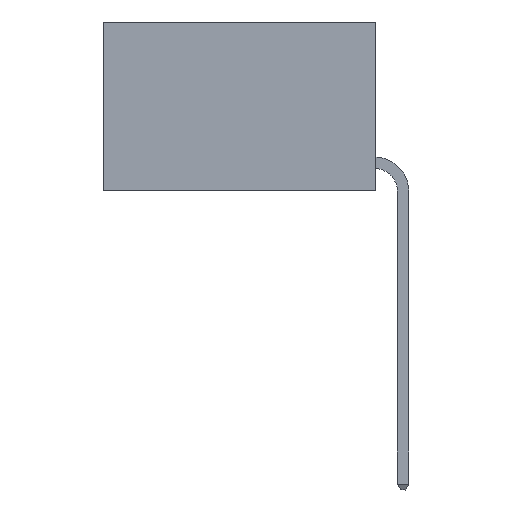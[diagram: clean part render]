
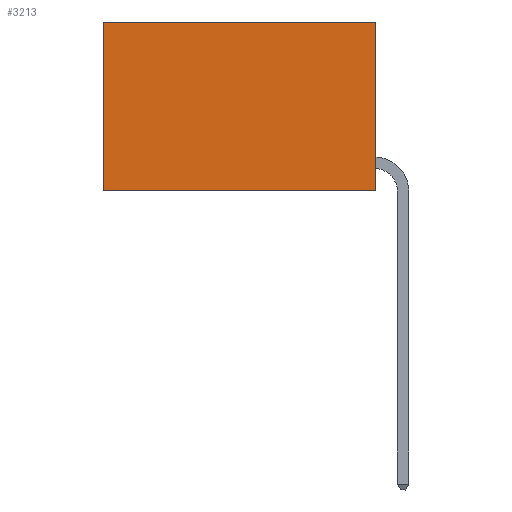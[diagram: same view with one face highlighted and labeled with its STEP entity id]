
A CAD part, left-side view. The second image highlights one B-rep face of the part: STEP entity #3213.
In plain terms, the highlighted planar face has unit normal (-1, 0, 0).
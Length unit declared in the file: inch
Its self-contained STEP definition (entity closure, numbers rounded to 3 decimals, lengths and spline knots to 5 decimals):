
#143 = LINE ( 'NONE', #2367, #5926 ) ;
#318 = ORIENTED_EDGE ( 'NONE', *, *, #11023, .F. ) ;
#419 = LINE ( 'NONE', #8445, #10663 ) ;
#1030 = VERTEX_POINT ( 'NONE', #12940 ) ;
#2367 = CARTESIAN_POINT ( 'NONE',  ( 0.2625, 0.6, 0. ) ) ;
#3051 = DIRECTION ( 'NONE',  ( 0., 0., -1. ) ) ;
#3123 = DIRECTION ( 'NONE',  ( 0., 1., 0. ) ) ;
#3213 = ADVANCED_FACE ( 'NONE', ( #9768 ), #10936, .F. ) ;
#3231 = ORIENTED_EDGE ( 'NONE', *, *, #10128, .T. ) ;
#4268 = ORIENTED_EDGE ( 'NONE', *, *, #4584, .T. ) ;
#4525 = CARTESIAN_POINT ( 'NONE',  ( 0.2625, 0., 0. ) ) ;
#4584 = EDGE_CURVE ( 'NONE', #11604, #11495, #143, .T. ) ;
#5003 = AXIS2_PLACEMENT_3D ( 'NONE', #4525, #6391, #5308 ) ;
#5061 = LINE ( 'NONE', #9364, #12695 ) ;
#5308 = DIRECTION ( 'NONE',  ( 0., 0., -1. ) ) ;
#5926 = VECTOR ( 'NONE', #6097, 39.37008 ) ;
#6097 = DIRECTION ( 'NONE',  ( 0., 0., -1. ) ) ;
#6391 = DIRECTION ( 'NONE',  ( 1., 0., 0. ) ) ;
#6423 = CARTESIAN_POINT ( 'NONE',  ( 0.2625, 0., -0.37 ) ) ;
#6830 = ORIENTED_EDGE ( 'NONE', *, *, #7465, .F. ) ;
#7410 = DIRECTION ( 'NONE',  ( 0., 1., 0. ) ) ;
#7465 = EDGE_CURVE ( 'NONE', #10747, #11495, #9661, .T. ) ;
#8074 = CARTESIAN_POINT ( 'NONE',  ( 0.2625, 0.6, -0.37 ) ) ;
#8445 = CARTESIAN_POINT ( 'NONE',  ( 0.2625, 0., 0. ) ) ;
#9364 = CARTESIAN_POINT ( 'NONE',  ( 0.2625, 0., 0. ) ) ;
#9661 = LINE ( 'NONE', #6423, #11768 ) ;
#9768 = FACE_OUTER_BOUND ( 'NONE', #11050, .T. ) ;
#10019 = CARTESIAN_POINT ( 'NONE',  ( 0.2625, 0.6, 0. ) ) ;
#10128 = EDGE_CURVE ( 'NONE', #1030, #11604, #5061, .T. ) ;
#10663 = VECTOR ( 'NONE', #3051, 39.37008 ) ;
#10747 = VERTEX_POINT ( 'NONE', #14018 ) ;
#10936 = PLANE ( 'NONE',  #5003 ) ;
#11023 = EDGE_CURVE ( 'NONE', #1030, #10747, #419, .T. ) ;
#11050 = EDGE_LOOP ( 'NONE', ( #4268, #6830, #318, #3231 ) ) ;
#11495 = VERTEX_POINT ( 'NONE', #8074 ) ;
#11604 = VERTEX_POINT ( 'NONE', #10019 ) ;
#11768 = VECTOR ( 'NONE', #3123, 39.37008 ) ;
#12695 = VECTOR ( 'NONE', #7410, 39.37008 ) ;
#12940 = CARTESIAN_POINT ( 'NONE',  ( 0.2625, 0., 0. ) ) ;
#14018 = CARTESIAN_POINT ( 'NONE',  ( 0.2625, 0., -0.37 ) ) ;
